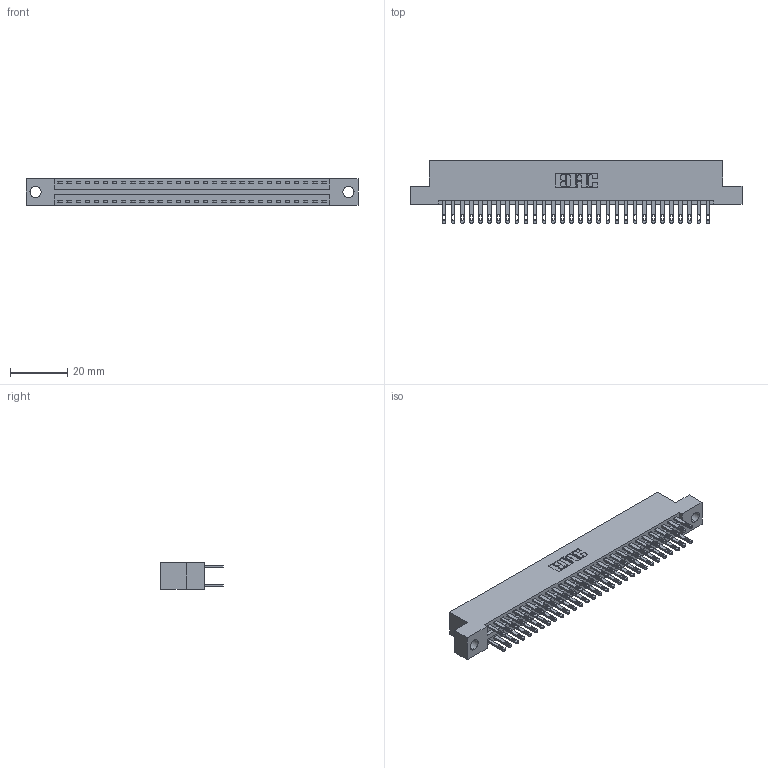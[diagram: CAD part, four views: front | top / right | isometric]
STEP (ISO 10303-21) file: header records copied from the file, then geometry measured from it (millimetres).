
FILE_DESCRIPTION (( 'STEP AP203' ), '1' );
FILE_NAME ('346-060-500-204.STEP', '2018-08-28T05:05:55', ( '' ), ( '' ), 'SwSTEP 2.0', 'SolidWorks 2016', '' );
FILE_SCHEMA (( 'CONFIG_CONTROL_DESIGN' ));
Length unit declared in the file: inch
Products named in the file (3): 346 Part_Flush Mounting Lugs - 0.156 Dia-TH; 345-292-001_345-293-100; 346-060-500-204
Assembly tree (61 placements, depth 2):
  346-060-500-204
    346 Part_Flush Mounting Lugs - 0.156 Dia-TH
    345-292-001_345-293-100  x60
Bounding box: 115.82 x 21.84 x 9.4 mm (x, y, z)
Volume: 11296.6 mm3; surface area: 15780.6 mm2
Topology: 61 solids, 61 shells, 3002 faces, 9149 edges, 6098 vertices
Faces by surface type: plane 1816, cylinder 1186
Entity records: 21127 total; most frequent: CARTESIAN_POINT 3496, ORIENTED_EDGE 3430, DIRECTION 3135, EDGE_CURVE 1715, VECTOR 1459, LINE 1459, VERTEX_POINT 1142, AXIS2_PLACEMENT_3D 838
